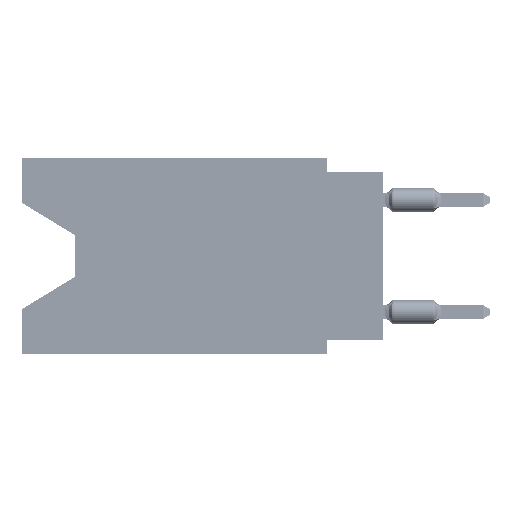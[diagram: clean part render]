
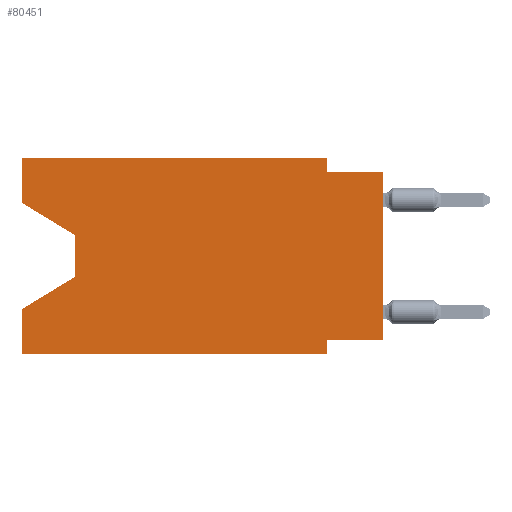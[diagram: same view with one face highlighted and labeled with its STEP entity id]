
A CAD part, left-side view. The second image highlights one B-rep face of the part: STEP entity #80451.
In plain terms, the highlighted planar face has unit normal (-1, 0, 0).
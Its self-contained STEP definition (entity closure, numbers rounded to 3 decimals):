
#1157 = DIRECTION ( 'NONE',  ( 0., 0., -1. ) ) ;
#1400 = CARTESIAN_POINT ( 'NONE',  ( 0., 2.54, -0.635 ) ) ;
#1664 = CARTESIAN_POINT ( 'NONE',  ( 0., 2.54, -8.89 ) ) ;
#2033 = CARTESIAN_POINT ( 'NONE',  ( 0., 13.97, -3.505 ) ) ;
#2139 = LINE ( 'NONE', #70530, #16371 ) ;
#2934 = EDGE_CURVE ( 'NONE', #55216, #35523, #2139, .T. ) ;
#5023 = CARTESIAN_POINT ( 'NONE',  ( 0., 16.383, 0. ) ) ;
#9515 = VERTEX_POINT ( 'NONE', #47338 ) ;
#10655 = VERTEX_POINT ( 'NONE', #66323 ) ;
#10993 = VECTOR ( 'NONE', #17960, 1000. ) ;
#11499 = PLANE ( 'NONE',  #90512 ) ;
#11745 = VERTEX_POINT ( 'NONE', #76274 ) ;
#13478 = LINE ( 'NONE', #40240, #36048 ) ;
#13856 = DIRECTION ( 'NONE',  ( 0., 0., 1. ) ) ;
#14201 = LINE ( 'NONE', #41422, #32256 ) ;
#14538 = CARTESIAN_POINT ( 'NONE',  ( 0., 0., -0.635 ) ) ;
#15830 = ORIENTED_EDGE ( 'NONE', *, *, #67555, .F. ) ;
#16353 = LINE ( 'NONE', #36190, #73808 ) ;
#16371 = VECTOR ( 'NONE', #51483, 1000. ) ;
#17535 = ORIENTED_EDGE ( 'NONE', *, *, #59558, .F. ) ;
#17960 = DIRECTION ( 'NONE',  ( 0., 0., 1. ) ) ;
#22708 = VECTOR ( 'NONE', #51386, 1000. ) ;
#26122 = CARTESIAN_POINT ( 'NONE',  ( 0., 13.97, -5.385 ) ) ;
#26235 = VECTOR ( 'NONE', #50513, 1000. ) ;
#26371 = VERTEX_POINT ( 'NONE', #1400 ) ;
#26901 = EDGE_CURVE ( 'NONE', #35523, #10655, #65204, .T. ) ;
#28906 = ORIENTED_EDGE ( 'NONE', *, *, #83076, .F. ) ;
#31422 = CARTESIAN_POINT ( 'NONE',  ( 0., 16.383, -8.89 ) ) ;
#32256 = VECTOR ( 'NONE', #42345, 1000. ) ;
#35250 = ORIENTED_EDGE ( 'NONE', *, *, #38798, .F. ) ;
#35523 = VERTEX_POINT ( 'NONE', #56615 ) ;
#35793 = VECTOR ( 'NONE', #73855, 1000. ) ;
#36048 = VECTOR ( 'NONE', #90470, 1000. ) ;
#36138 = ORIENTED_EDGE ( 'NONE', *, *, #81514, .T. ) ;
#36190 = CARTESIAN_POINT ( 'NONE',  ( 0., 2.54, 0. ) ) ;
#36284 = CARTESIAN_POINT ( 'NONE',  ( 0., 0., -0.635 ) ) ;
#36705 = LINE ( 'NONE', #1664, #26235 ) ;
#38798 = EDGE_CURVE ( 'NONE', #26371, #84072, #84180, .T. ) ;
#40240 = CARTESIAN_POINT ( 'NONE',  ( 0., 0., -8.255 ) ) ;
#41159 = VERTEX_POINT ( 'NONE', #87228 ) ;
#41422 = CARTESIAN_POINT ( 'NONE',  ( 0., 16.383, 0. ) ) ;
#41742 = VERTEX_POINT ( 'NONE', #75542 ) ;
#42345 = DIRECTION ( 'NONE',  ( 0., -1., 0. ) ) ;
#42675 = DIRECTION ( 'NONE',  ( 0., -1., 0. ) ) ;
#42901 = CARTESIAN_POINT ( 'NONE',  ( 0., 16.383, 0. ) ) ;
#45057 = VERTEX_POINT ( 'NONE', #45561 ) ;
#45485 = CARTESIAN_POINT ( 'NONE',  ( 0., 2.54, 0. ) ) ;
#45561 = CARTESIAN_POINT ( 'NONE',  ( 0., 16.383, -6.852 ) ) ;
#46545 = DIRECTION ( 'NONE',  ( 1., 0., 0. ) ) ;
#46809 = ORIENTED_EDGE ( 'NONE', *, *, #61629, .T. ) ;
#47331 = EDGE_CURVE ( 'NONE', #10655, #45057, #61167, .T. ) ;
#47338 = CARTESIAN_POINT ( 'NONE',  ( 0., 2.54, -8.89 ) ) ;
#47428 = FACE_OUTER_BOUND ( 'NONE', #75865, .T. ) ;
#47887 = LINE ( 'NONE', #5023, #10993 ) ;
#49079 = ORIENTED_EDGE ( 'NONE', *, *, #2934, .T. ) ;
#49967 = CARTESIAN_POINT ( 'NONE',  ( 0., 16.383, -8.89 ) ) ;
#50513 = DIRECTION ( 'NONE',  ( 0., 0., -1. ) ) ;
#51386 = DIRECTION ( 'NONE',  ( 0., 0., -1. ) ) ;
#51483 = DIRECTION ( 'NONE',  ( 0., -0.855, -0.519 ) ) ;
#52868 = VERTEX_POINT ( 'NONE', #49967 ) ;
#55216 = VERTEX_POINT ( 'NONE', #72784 ) ;
#55308 = ORIENTED_EDGE ( 'NONE', *, *, #47331, .T. ) ;
#55987 = ORIENTED_EDGE ( 'NONE', *, *, #59164, .F. ) ;
#56117 = ORIENTED_EDGE ( 'NONE', *, *, #80515, .F. ) ;
#56615 = CARTESIAN_POINT ( 'NONE',  ( 0., 13.97, -3.505 ) ) ;
#59164 = EDGE_CURVE ( 'NONE', #86320, #26371, #16353, .T. ) ;
#59558 = EDGE_CURVE ( 'NONE', #55216, #11745, #77026, .T. ) ;
#59715 = VECTOR ( 'NONE', #89660, 1000. ) ;
#59936 = DIRECTION ( 'NONE',  ( 0., 0., -1. ) ) ;
#60579 = VECTOR ( 'NONE', #13856, 1000. ) ;
#61167 = LINE ( 'NONE', #26122, #82766 ) ;
#61295 = CARTESIAN_POINT ( 'NONE',  ( 0., 16.383, 0. ) ) ;
#61629 = EDGE_CURVE ( 'NONE', #52868, #9515, #66475, .T. ) ;
#61991 = CARTESIAN_POINT ( 'NONE',  ( 0., 0., 0. ) ) ;
#64015 = VECTOR ( 'NONE', #42675, 1000. ) ;
#65204 = LINE ( 'NONE', #2033, #22708 ) ;
#66323 = CARTESIAN_POINT ( 'NONE',  ( 0., 13.97, -5.385 ) ) ;
#66475 = LINE ( 'NONE', #31422, #35793 ) ;
#67555 = EDGE_CURVE ( 'NONE', #41742, #9515, #36705, .T. ) ;
#69441 = DIRECTION ( 'NONE',  ( 0., 0.855, -0.519 ) ) ;
#70530 = CARTESIAN_POINT ( 'NONE',  ( 0., 16.383, -2.038 ) ) ;
#72784 = CARTESIAN_POINT ( 'NONE',  ( 0., 16.383, -2.038 ) ) ;
#73540 = EDGE_CURVE ( 'NONE', #11745, #86320, #14201, .T. ) ;
#73808 = VECTOR ( 'NONE', #1157, 1000. ) ;
#73855 = DIRECTION ( 'NONE',  ( 0., -1., 0. ) ) ;
#74707 = ORIENTED_EDGE ( 'NONE', *, *, #26901, .T. ) ;
#75369 = LINE ( 'NONE', #61991, #59715 ) ;
#75542 = CARTESIAN_POINT ( 'NONE',  ( 0., 2.54, -8.255 ) ) ;
#75865 = EDGE_LOOP ( 'NONE', ( #49079, #74707, #55308, #56117, #46809, #15830, #28906, #36138, #35250, #55987, #76965, #17535 ) ) ;
#76274 = CARTESIAN_POINT ( 'NONE',  ( 0., 16.383, 0. ) ) ;
#76965 = ORIENTED_EDGE ( 'NONE', *, *, #73540, .F. ) ;
#77026 = LINE ( 'NONE', #42901, #60579 ) ;
#80451 = ADVANCED_FACE ( 'NONE', ( #47428 ), #11499, .F. ) ;
#80515 = EDGE_CURVE ( 'NONE', #52868, #45057, #47887, .T. ) ;
#81514 = EDGE_CURVE ( 'NONE', #41159, #84072, #75369, .T. ) ;
#82766 = VECTOR ( 'NONE', #69441, 1000. ) ;
#83076 = EDGE_CURVE ( 'NONE', #41159, #41742, #13478, .T. ) ;
#84072 = VERTEX_POINT ( 'NONE', #36284 ) ;
#84180 = LINE ( 'NONE', #14538, #64015 ) ;
#86320 = VERTEX_POINT ( 'NONE', #45485 ) ;
#87228 = CARTESIAN_POINT ( 'NONE',  ( 0., 0., -8.255 ) ) ;
#89660 = DIRECTION ( 'NONE',  ( 0., 0., 1. ) ) ;
#90470 = DIRECTION ( 'NONE',  ( 0., 1., 0. ) ) ;
#90512 = AXIS2_PLACEMENT_3D ( 'NONE', #61295, #46545, #59936 ) ;
